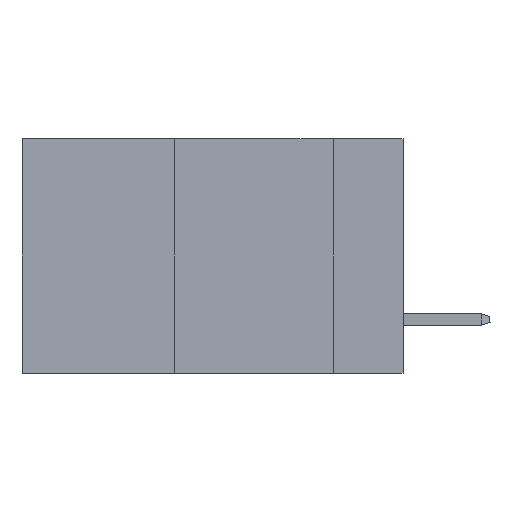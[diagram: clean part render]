
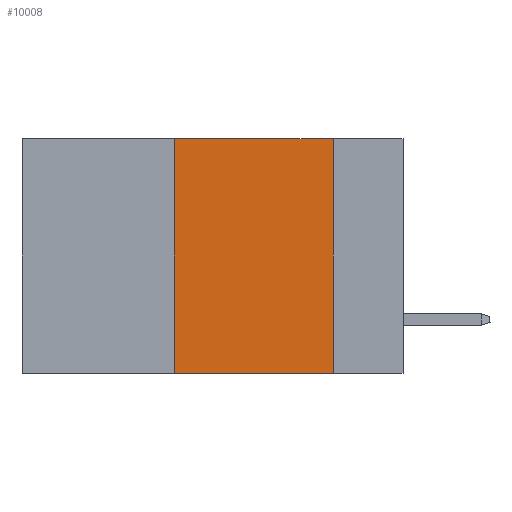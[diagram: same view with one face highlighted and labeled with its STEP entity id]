
A CAD part, left-side view. The second image highlights one B-rep face of the part: STEP entity #10008.
In plain terms, the highlighted planar face has unit normal (-1, 0, 0).
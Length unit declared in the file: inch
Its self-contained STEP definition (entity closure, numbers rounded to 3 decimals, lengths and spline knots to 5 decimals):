
#471 = CARTESIAN_POINT ( 'NONE',  ( 0., 0.36, -0.37 ) ) ;
#835 = EDGE_CURVE ( 'NONE', #18751, #7936, #1597, .T. ) ;
#1597 = LINE ( 'NONE', #3036, #9178 ) ;
#1599 = CARTESIAN_POINT ( 'NONE',  ( 0., 0.6, 0. ) ) ;
#1785 = CARTESIAN_POINT ( 'NONE',  ( 0., 0.11, -0.37 ) ) ;
#3036 = CARTESIAN_POINT ( 'NONE',  ( 0., 0.36, 0. ) ) ;
#3782 = DIRECTION ( 'NONE',  ( 0., 0., -1. ) ) ;
#3958 = CARTESIAN_POINT ( 'NONE',  ( 0., 0.6, 0. ) ) ;
#5198 = AXIS2_PLACEMENT_3D ( 'NONE', #1599, #15146, #16981 ) ;
#6231 = EDGE_CURVE ( 'NONE', #18751, #13374, #18701, .T. ) ;
#6282 = DIRECTION ( 'NONE',  ( 0., 0., 1. ) ) ;
#7521 = CARTESIAN_POINT ( 'NONE',  ( 0., 0.11, 0. ) ) ;
#7936 = VERTEX_POINT ( 'NONE', #11696 ) ;
#8181 = VECTOR ( 'NONE', #16290, 39.37008 ) ;
#9104 = FACE_OUTER_BOUND ( 'NONE', #15845, .T. ) ;
#9178 = VECTOR ( 'NONE', #6282, 39.37008 ) ;
#9212 = DIRECTION ( 'NONE',  ( 0., -1., 0. ) ) ;
#9489 = EDGE_CURVE ( 'NONE', #7936, #10786, #17798, .T. ) ;
#10008 = ADVANCED_FACE ( 'NONE', ( #9104 ), #13637, .F. ) ;
#10309 = VECTOR ( 'NONE', #9212, 39.37008 ) ;
#10786 = VERTEX_POINT ( 'NONE', #7521 ) ;
#11479 = LINE ( 'NONE', #17631, #14133 ) ;
#11696 = CARTESIAN_POINT ( 'NONE',  ( 0., 0.36, 0. ) ) ;
#12069 = EDGE_CURVE ( 'NONE', #10786, #13374, #11479, .T. ) ;
#13081 = ORIENTED_EDGE ( 'NONE', *, *, #6231, .T. ) ;
#13374 = VERTEX_POINT ( 'NONE', #1785 ) ;
#13637 = PLANE ( 'NONE',  #5198 ) ;
#14133 = VECTOR ( 'NONE', #3782, 39.37008 ) ;
#14513 = ORIENTED_EDGE ( 'NONE', *, *, #12069, .F. ) ;
#15146 = DIRECTION ( 'NONE',  ( 1., 0., 0. ) ) ;
#15147 = ORIENTED_EDGE ( 'NONE', *, *, #9489, .F. ) ;
#15347 = CARTESIAN_POINT ( 'NONE',  ( 0., 0.6, -0.37 ) ) ;
#15845 = EDGE_LOOP ( 'NONE', ( #14513, #15147, #18601, #13081 ) ) ;
#16290 = DIRECTION ( 'NONE',  ( 0., -1., 0. ) ) ;
#16981 = DIRECTION ( 'NONE',  ( 0., 0., -1. ) ) ;
#17631 = CARTESIAN_POINT ( 'NONE',  ( 0., 0.11, 0. ) ) ;
#17798 = LINE ( 'NONE', #3958, #8181 ) ;
#18601 = ORIENTED_EDGE ( 'NONE', *, *, #835, .F. ) ;
#18701 = LINE ( 'NONE', #15347, #10309 ) ;
#18751 = VERTEX_POINT ( 'NONE', #471 ) ;
